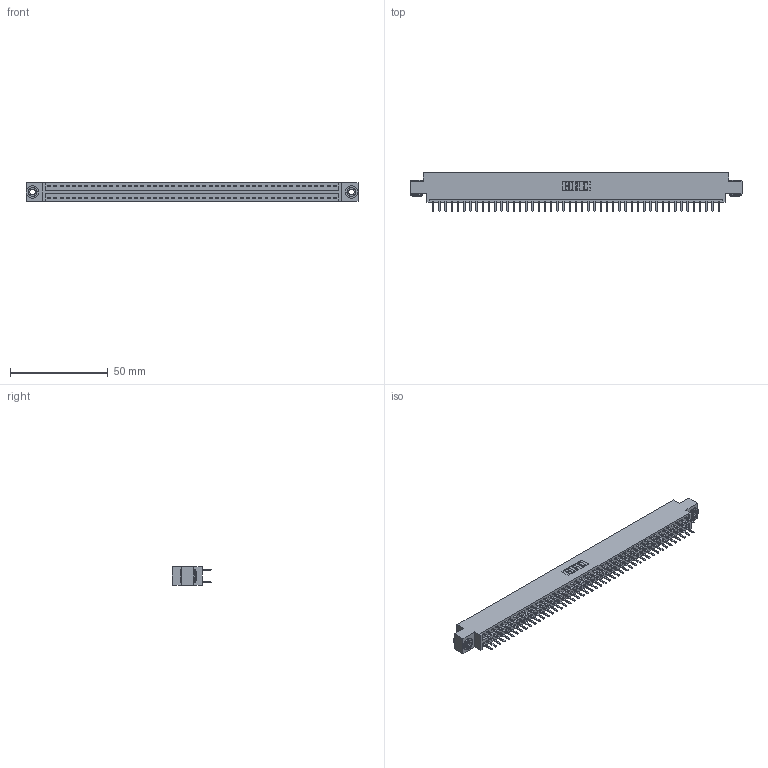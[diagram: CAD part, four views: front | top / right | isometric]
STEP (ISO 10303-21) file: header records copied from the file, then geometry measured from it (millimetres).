
FILE_DESCRIPTION (( 'STEP AP203' ), '1' );
FILE_NAME ('346-094-520-803.STEP', '2022-05-26T09:26:19', ( '' ), ( '' ), 'SwSTEP 2.0', 'SolidWorks 2020', '' );
FILE_SCHEMA (( 'CONFIG_CONTROL_DESIGN' ));
Length unit declared in the file: inch
Products named in the file (4): 345-250-002_345-250-002-102; 346 Part_0.170 Offset - 0.156 Dia-TH; 345-292-001_345-293-120; 346-094-520-803
Assembly tree (97 placements, depth 2):
  346-094-520-803
    346 Part_0.170 Offset - 0.156 Dia-TH
    345-292-001_345-293-120  x94
    345-250-002_345-250-002-102  x2
Bounding box: 169.8 x 20.02 x 9.4 mm (x, y, z)
Volume: 16401.7 mm3; surface area: 22955.4 mm2
Topology: 97 solids, 97 shells, 5442 faces, 15775 edges, 10262 vertices
Faces by surface type: plane 3582, cylinder 1852, cone 8
Entity records: 31312 total; most frequent: CARTESIAN_POINT 5149, ORIENTED_EDGE 5062, DIRECTION 4605, EDGE_CURVE 2531, LINE 2183, VECTOR 2183, VERTEX_POINT 1682, AXIS2_PLACEMENT_3D 1211
